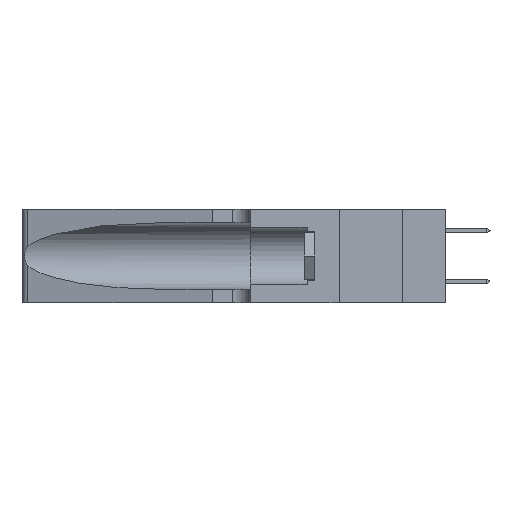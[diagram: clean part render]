
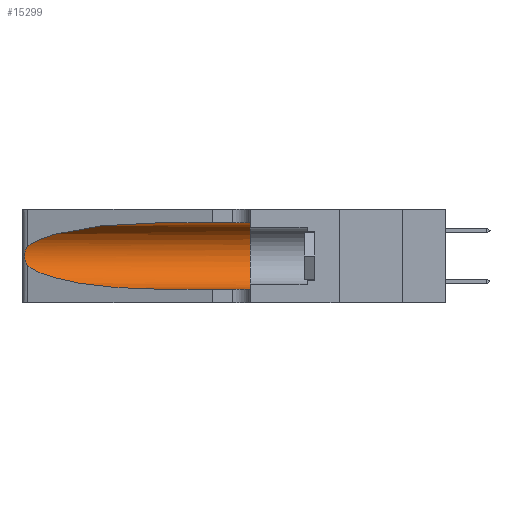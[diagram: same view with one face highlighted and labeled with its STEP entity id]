
A CAD part, left-side view. The second image highlights one B-rep face of the part: STEP entity #15299.
In plain terms, the highlighted cylindrical face has radius 3.308 mm (diameter 6.617 mm), a partial arc.
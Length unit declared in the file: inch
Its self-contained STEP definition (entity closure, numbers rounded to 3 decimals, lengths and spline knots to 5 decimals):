
#1129 = DIRECTION ( 'NONE',  ( 0., 0., -1. ) ) ;
#1540 = CARTESIAN_POINT ( 'NONE',  ( 0.26017, 1.23833, 0.17102 ) ) ;
#3266 = EDGE_CURVE ( 'NONE', #17437, #13514, #10143, .T. ) ;
#3376 = CARTESIAN_POINT ( 'NONE',  ( 0.1305, 0.72297, 0.05475 ) ) ;
#3474 = ORIENTED_EDGE ( 'NONE', *, *, #10951, .F. ) ;
#3777 = CARTESIAN_POINT ( 'NONE',  ( 0.25789, 1.23486, 0.15765 ) ) ;
#4932 = CARTESIAN_POINT ( 'NONE',  ( 0.1305, 0.72297, 0.31525 ) ) ;
#5260 = DIRECTION ( 'NONE',  ( 0., -1., 0. ) ) ;
#5455 = CARTESIAN_POINT ( 'NONE',  ( 0.18966, 0.96281, 0.05475 ) ) ;
#5551 = CARTESIAN_POINT ( 'NONE',  ( 0.1305, 0.72297, 0.05475 ) ) ;
#6043 = CARTESIAN_POINT ( 'NONE',  ( 0.25555, 1.22993, 0.14849 ) ) ;
#6146 = DIRECTION ( 'NONE',  ( 0., 1., 0. ) ) ;
#6292 = CARTESIAN_POINT ( 'NONE',  ( 0.1305, 0.35, 0.31525 ) ) ;
#6729 = DIRECTION ( 'NONE',  ( 0., -1., 0. ) ) ;
#7208 = CARTESIAN_POINT ( 'NONE',  ( 0.18966, 0.96281, 0.31525 ) ) ;
#8284 = CYLINDRICAL_SURFACE ( 'NONE', #12205, 0.13025 ) ;
#8544 = AXIS2_PLACEMENT_3D ( 'NONE', #19512, #6146, #21755 ) ;
#8683 = LINE ( 'NONE', #9827, #26454 ) ;
#8954 = ORIENTED_EDGE ( 'NONE', *, *, #3266, .T. ) ;
#8990 = FACE_OUTER_BOUND ( 'NONE', #17588, .T. ) ;
#9497 = CARTESIAN_POINT ( 'NONE',  ( 0.25487, 1.22718, 0.22369 ) ) ;
#9827 = CARTESIAN_POINT ( 'NONE',  ( 0.1305, 1.61858, 0.31525 ) ) ;
#10143 =( BOUNDED_CURVE ( )  B_SPLINE_CURVE ( 3, ( #18907, #27798, #5455, #5551 ),
 .UNSPECIFIED., .F., .T. ) 
 B_SPLINE_CURVE_WITH_KNOTS ( ( 4, 4 ),
 ( 3.44316, 4.71239 ),
 .UNSPECIFIED. ) 
 CURVE ( )  GEOMETRIC_REPRESENTATION_ITEM ( )  RATIONAL_B_SPLINE_CURVE ( ( 1., 0.87, 0.87, 1. ) ) 
 REPRESENTATION_ITEM ( '' )  );
#10253 = EDGE_CURVE ( 'NONE', #23873, #21936, #25445, .T. ) ;
#10536 = CARTESIAN_POINT ( 'NONE',  ( 0.25787, 1.23484, 0.2124 ) ) ;
#10951 = EDGE_CURVE ( 'NONE', #25249, #23873, #8683, .T. ) ;
#11046 = B_SPLINE_CURVE_WITH_KNOTS ( 'NONE', 3,
 ( #21566, #19322, #23812, #10536, #26063, #12745, #28282, #14984, #1540, #17198, #3777, #19420, #6043, #21660 ),
 .UNSPECIFIED., .F., .F.,
 ( 4, 2, 2, 2, 2, 2, 4 ),
 ( 0., 0.00027, 0.00053, 0.00107, 0.0016, 0.00187, 0.00214 ),
 .UNSPECIFIED. ) ;
#11997 = ORIENTED_EDGE ( 'NONE', *, *, #26378, .T. ) ;
#12205 = AXIS2_PLACEMENT_3D ( 'NONE', #25646, #12346, #1129 ) ;
#12346 = DIRECTION ( 'NONE',  ( 0., -1., 0. ) ) ;
#12745 = CARTESIAN_POINT ( 'NONE',  ( 0.26018, 1.23835, 0.19895 ) ) ;
#13316 = CARTESIAN_POINT ( 'NONE',  ( 0.1305, 0.72297, 0.31525 ) ) ;
#13514 = VERTEX_POINT ( 'NONE', #3376 ) ;
#13522 = CARTESIAN_POINT ( 'NONE',  ( 0.1305, 1.61858, 0.05475 ) ) ;
#13953 = CARTESIAN_POINT ( 'NONE',  ( 0.25487, 1.22718, 0.14631 ) ) ;
#14012 = VECTOR ( 'NONE', #6729, 39.37008 ) ;
#14984 = CARTESIAN_POINT ( 'NONE',  ( 0.26075, 1.23896, 0.178 ) ) ;
#15299 = ADVANCED_FACE ( 'NONE', ( #8990 ), #8284, .F. ) ;
#16745 = VERTEX_POINT ( 'NONE', #20375 ) ;
#16780 = EDGE_CURVE ( 'NONE', #25249, #16745, #21326, .T. ) ;
#17198 = CARTESIAN_POINT ( 'NONE',  ( 0.25856, 1.23593, 0.16098 ) ) ;
#17437 = VERTEX_POINT ( 'NONE', #13953 ) ;
#17588 = EDGE_LOOP ( 'NONE', ( #27104, #28479, #8954, #11997, #18196, #3474 ) ) ;
#18196 = ORIENTED_EDGE ( 'NONE', *, *, #10253, .F. ) ;
#18346 = EDGE_CURVE ( 'NONE', #16745, #17437, #11046, .T. ) ;
#18907 = CARTESIAN_POINT ( 'NONE',  ( 0.25487, 1.22718, 0.14631 ) ) ;
#19322 = CARTESIAN_POINT ( 'NONE',  ( 0.25555, 1.22994, 0.2215 ) ) ;
#19420 = CARTESIAN_POINT ( 'NONE',  ( 0.25639, 1.23186, 0.15144 ) ) ;
#19512 = CARTESIAN_POINT ( 'NONE',  ( 0.1305, 0.35, 0.185 ) ) ;
#20375 = CARTESIAN_POINT ( 'NONE',  ( 0.25487, 1.22718, 0.22369 ) ) ;
#21326 =( BOUNDED_CURVE ( )  B_SPLINE_CURVE ( 3, ( #4932, #7208, #22805, #9497 ),
 .UNSPECIFIED., .F., .T. ) 
 B_SPLINE_CURVE_WITH_KNOTS ( ( 4, 4 ),
 ( 1.5708, 2.84003 ),
 .UNSPECIFIED. ) 
 CURVE ( )  GEOMETRIC_REPRESENTATION_ITEM ( )  RATIONAL_B_SPLINE_CURVE ( ( 1., 0.87, 0.87, 1. ) ) 
 REPRESENTATION_ITEM ( '' )  );
#21566 = CARTESIAN_POINT ( 'NONE',  ( 0.25487, 1.22718, 0.22369 ) ) ;
#21660 = CARTESIAN_POINT ( 'NONE',  ( 0.25487, 1.22718, 0.14631 ) ) ;
#21755 = DIRECTION ( 'NONE',  ( 0., 0., 1. ) ) ;
#21936 = VERTEX_POINT ( 'NONE', #26088 ) ;
#22805 = CARTESIAN_POINT ( 'NONE',  ( 0.2373, 1.15595, 0.28018 ) ) ;
#23812 = CARTESIAN_POINT ( 'NONE',  ( 0.25639, 1.23184, 0.21858 ) ) ;
#23873 = VERTEX_POINT ( 'NONE', #6292 ) ;
#25249 = VERTEX_POINT ( 'NONE', #13316 ) ;
#25445 = CIRCLE ( 'NONE', #8544, 0.13025 ) ;
#25646 = CARTESIAN_POINT ( 'NONE',  ( 0.1305, 1.61858, 0.185 ) ) ;
#25833 = LINE ( 'NONE', #13522, #14012 ) ;
#26063 = CARTESIAN_POINT ( 'NONE',  ( 0.25854, 1.2359, 0.20912 ) ) ;
#26088 = CARTESIAN_POINT ( 'NONE',  ( 0.1305, 0.35, 0.05475 ) ) ;
#26378 = EDGE_CURVE ( 'NONE', #13514, #21936, #25833, .T. ) ;
#26454 = VECTOR ( 'NONE', #5260, 39.37008 ) ;
#27104 = ORIENTED_EDGE ( 'NONE', *, *, #16780, .T. ) ;
#27798 = CARTESIAN_POINT ( 'NONE',  ( 0.2373, 1.15595, 0.08982 ) ) ;
#28282 = CARTESIAN_POINT ( 'NONE',  ( 0.26075, 1.23896, 0.19203 ) ) ;
#28479 = ORIENTED_EDGE ( 'NONE', *, *, #18346, .T. ) ;
